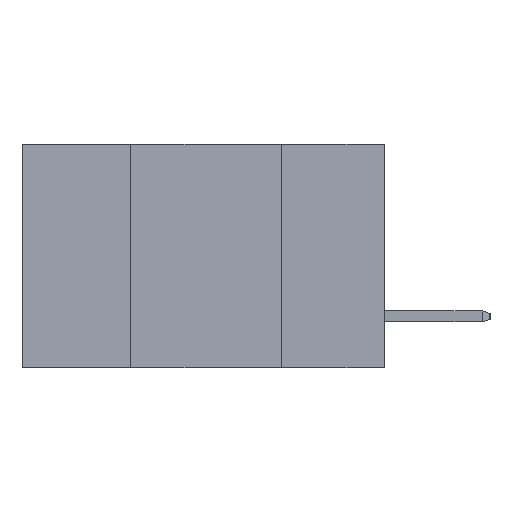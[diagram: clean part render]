
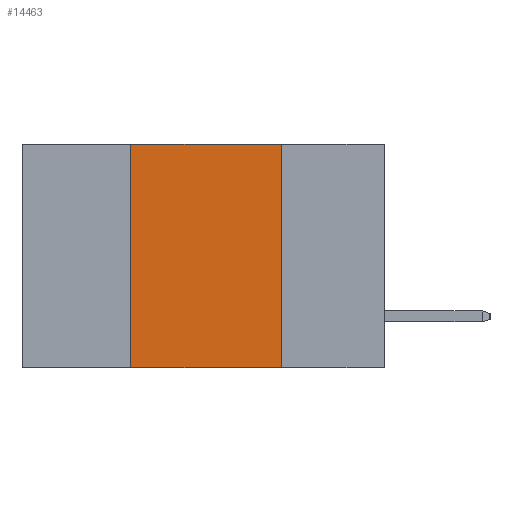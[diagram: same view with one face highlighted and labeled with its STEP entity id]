
A CAD part, left-side view. The second image highlights one B-rep face of the part: STEP entity #14463.
In plain terms, the highlighted planar face has unit normal (-1, 0, 0).
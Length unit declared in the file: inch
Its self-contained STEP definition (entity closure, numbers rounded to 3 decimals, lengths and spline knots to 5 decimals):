
#913 = ORIENTED_EDGE ( 'NONE', *, *, #17266, .F. ) ;
#1101 = CARTESIAN_POINT ( 'NONE',  ( 0., 0.17, 0. ) ) ;
#2222 = LINE ( 'NONE', #13786, #19837 ) ;
#2224 = CARTESIAN_POINT ( 'NONE',  ( 0., 0.6, 0. ) ) ;
#3426 = VERTEX_POINT ( 'NONE', #14297 ) ;
#5311 = LINE ( 'NONE', #12312, #10515 ) ;
#6059 = VERTEX_POINT ( 'NONE', #18238 ) ;
#6317 = DIRECTION ( 'NONE',  ( 0., 0., -1. ) ) ;
#6460 = DIRECTION ( 'NONE',  ( 1., 0., 0. ) ) ;
#6467 = CARTESIAN_POINT ( 'NONE',  ( 0., 0.6, 0. ) ) ;
#6810 = FACE_OUTER_BOUND ( 'NONE', #15042, .T. ) ;
#6993 = PLANE ( 'NONE',  #18842 ) ;
#7276 = EDGE_CURVE ( 'NONE', #3426, #15115, #5311, .T. ) ;
#8549 = VECTOR ( 'NONE', #20768, 39.37008 ) ;
#9133 = ORIENTED_EDGE ( 'NONE', *, *, #9604, .T. ) ;
#9604 = EDGE_CURVE ( 'NONE', #3426, #6059, #2222, .T. ) ;
#10456 = VERTEX_POINT ( 'NONE', #1101 ) ;
#10515 = VECTOR ( 'NONE', #12308, 39.37008 ) ;
#12308 = DIRECTION ( 'NONE',  ( 0., 0., 1. ) ) ;
#12312 = CARTESIAN_POINT ( 'NONE',  ( 0., 0.42, -0.37 ) ) ;
#13739 = DIRECTION ( 'NONE',  ( 0., -1., 0. ) ) ;
#13786 = CARTESIAN_POINT ( 'NONE',  ( 0., 0.6, -0.37 ) ) ;
#14297 = CARTESIAN_POINT ( 'NONE',  ( 0., 0.42, -0.37 ) ) ;
#14463 = ADVANCED_FACE ( 'NONE', ( #6810 ), #6993, .F. ) ;
#15042 = EDGE_LOOP ( 'NONE', ( #15850, #913, #20166, #9133 ) ) ;
#15115 = VERTEX_POINT ( 'NONE', #17996 ) ;
#15850 = ORIENTED_EDGE ( 'NONE', *, *, #18493, .F. ) ;
#17266 = EDGE_CURVE ( 'NONE', #15115, #10456, #18394, .T. ) ;
#17503 = CARTESIAN_POINT ( 'NONE',  ( 0., 0.17, -0.37 ) ) ;
#17694 = DIRECTION ( 'NONE',  ( 0., -1., 0. ) ) ;
#17890 = VECTOR ( 'NONE', #17694, 39.37008 ) ;
#17996 = CARTESIAN_POINT ( 'NONE',  ( 0., 0.42, 0. ) ) ;
#18238 = CARTESIAN_POINT ( 'NONE',  ( 0., 0.17, -0.37 ) ) ;
#18394 = LINE ( 'NONE', #2224, #17890 ) ;
#18493 = EDGE_CURVE ( 'NONE', #10456, #6059, #21881, .T. ) ;
#18842 = AXIS2_PLACEMENT_3D ( 'NONE', #6467, #6460, #6317 ) ;
#19837 = VECTOR ( 'NONE', #13739, 39.37008 ) ;
#20166 = ORIENTED_EDGE ( 'NONE', *, *, #7276, .F. ) ;
#20768 = DIRECTION ( 'NONE',  ( 0., 0., -1. ) ) ;
#21881 = LINE ( 'NONE', #17503, #8549 ) ;
